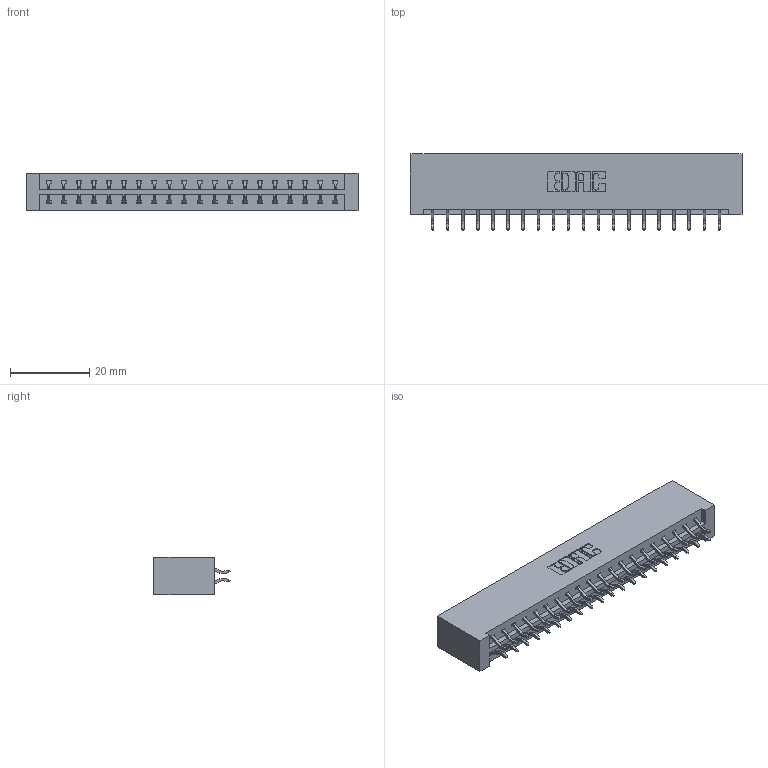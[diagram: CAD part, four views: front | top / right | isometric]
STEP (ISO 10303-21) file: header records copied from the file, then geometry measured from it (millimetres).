
FILE_DESCRIPTION (( 'STEP AP203' ), '1' );
FILE_NAME ('379-040-556-201.STEP', '2020-02-26T17:16:53', ( '' ), ( '' ), 'SwSTEP 2.0', 'SolidWorks 2016', '' );
FILE_SCHEMA (( 'CONFIG_CONTROL_DESIGN' ));
Length unit declared in the file: inch
Products named in the file (3): 379 Part_Lugless; 345-292-001_556 Tail; 379-040-556-201
Assembly tree (41 placements, depth 2):
  379-040-556-201
    379 Part_Lugless
    345-292-001_556 Tail  x40
Bounding box: 83.82 x 19.24 x 9.53 mm (x, y, z)
Volume: 9393.7 mm3; surface area: 10347 mm2
Topology: 41 solids, 41 shells, 2426 faces, 7207 edges, 4750 vertices
Faces by surface type: plane 1666, cylinder 760
Entity records: 15655 total; most frequent: CARTESIAN_POINT 2634, ORIENTED_EDGE 2558, DIRECTION 2271, EDGE_CURVE 1279, VECTOR 1151, LINE 1151, VERTEX_POINT 850, AXIS2_PLACEMENT_3D 560
